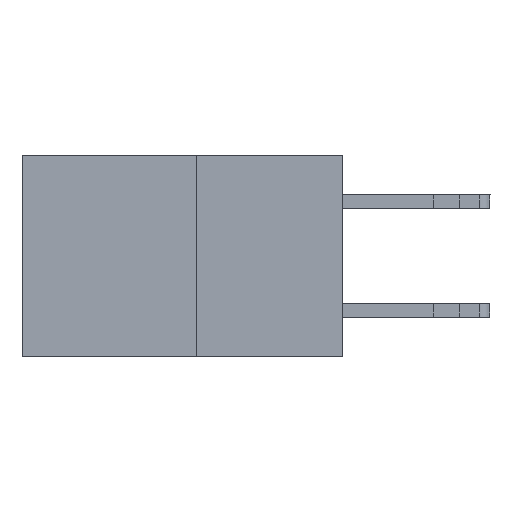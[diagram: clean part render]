
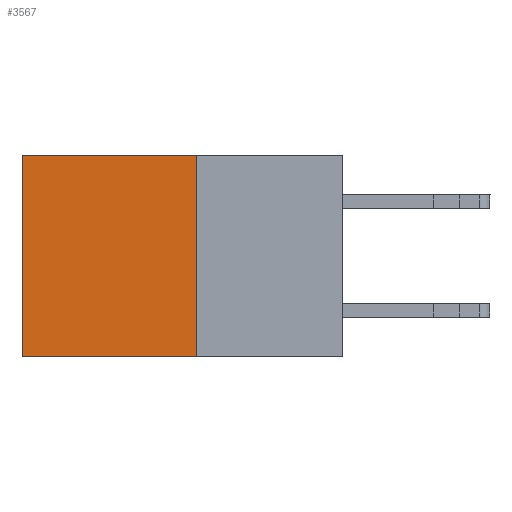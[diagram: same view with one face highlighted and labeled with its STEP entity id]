
A CAD part, left-side view. The second image highlights one B-rep face of the part: STEP entity #3567.
In plain terms, the highlighted planar face has unit normal (-1, 0, 0).
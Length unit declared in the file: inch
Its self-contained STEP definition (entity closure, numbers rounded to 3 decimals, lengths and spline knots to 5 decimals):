
#103 = VERTEX_POINT ( 'NONE', #18160 ) ;
#352 = LINE ( 'NONE', #631, #13703 ) ;
#631 = CARTESIAN_POINT ( 'NONE',  ( 0.277, 0.27, 0. ) ) ;
#1267 = DIRECTION ( 'NONE',  ( 0., 0., -1. ) ) ;
#2110 = VERTEX_POINT ( 'NONE', #2735 ) ;
#2573 = EDGE_CURVE ( 'NONE', #103, #2110, #15072, .T. ) ;
#2735 = CARTESIAN_POINT ( 'NONE',  ( 0.277, 0.59, -0.37 ) ) ;
#2886 = CARTESIAN_POINT ( 'NONE',  ( 0.277, 0.27, -0.37 ) ) ;
#3281 = DIRECTION ( 'NONE',  ( 0., 0., -1. ) ) ;
#3567 = ADVANCED_FACE ( 'NONE', ( #18185 ), #9971, .F. ) ;
#4202 = CARTESIAN_POINT ( 'NONE',  ( 0.277, 0.27, -0.37 ) ) ;
#4413 = LINE ( 'NONE', #14291, #11292 ) ;
#4737 = ORIENTED_EDGE ( 'NONE', *, *, #2573, .T. ) ;
#5924 = VECTOR ( 'NONE', #9985, 39.37008 ) ;
#6237 = DIRECTION ( 'NONE',  ( 0., 1., 0. ) ) ;
#7082 = ORIENTED_EDGE ( 'NONE', *, *, #17698, .F. ) ;
#7838 = CARTESIAN_POINT ( 'NONE',  ( 0.277, 0.59, -0.37 ) ) ;
#7951 = EDGE_LOOP ( 'NONE', ( #4737, #7082, #11794, #15994 ) ) ;
#8175 = CARTESIAN_POINT ( 'NONE',  ( 0.277, 0.27, -0.37 ) ) ;
#8366 = VERTEX_POINT ( 'NONE', #17393 ) ;
#9878 = DIRECTION ( 'NONE',  ( 1., 0., 0. ) ) ;
#9971 = PLANE ( 'NONE',  #10196 ) ;
#9978 = VECTOR ( 'NONE', #3281, 39.37008 ) ;
#9985 = DIRECTION ( 'NONE',  ( 0., 1., 0. ) ) ;
#10196 = AXIS2_PLACEMENT_3D ( 'NONE', #8175, #9878, #15592 ) ;
#10279 = LINE ( 'NONE', #4202, #5924 ) ;
#11292 = VECTOR ( 'NONE', #1267, 39.37008 ) ;
#11794 = ORIENTED_EDGE ( 'NONE', *, *, #12268, .F. ) ;
#12064 = EDGE_CURVE ( 'NONE', #8366, #103, #352, .T. ) ;
#12268 = EDGE_CURVE ( 'NONE', #8366, #18699, #4413, .T. ) ;
#13703 = VECTOR ( 'NONE', #6237, 39.37008 ) ;
#14291 = CARTESIAN_POINT ( 'NONE',  ( 0.277, 0.27, -0.37 ) ) ;
#15072 = LINE ( 'NONE', #7838, #9978 ) ;
#15592 = DIRECTION ( 'NONE',  ( 0., 0., -1. ) ) ;
#15994 = ORIENTED_EDGE ( 'NONE', *, *, #12064, .T. ) ;
#17393 = CARTESIAN_POINT ( 'NONE',  ( 0.277, 0.27, 0. ) ) ;
#17698 = EDGE_CURVE ( 'NONE', #18699, #2110, #10279, .T. ) ;
#18160 = CARTESIAN_POINT ( 'NONE',  ( 0.277, 0.59, 0. ) ) ;
#18185 = FACE_OUTER_BOUND ( 'NONE', #7951, .T. ) ;
#18699 = VERTEX_POINT ( 'NONE', #2886 ) ;
